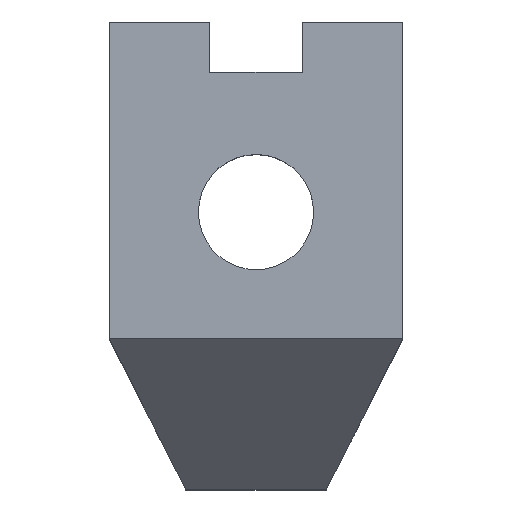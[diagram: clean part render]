
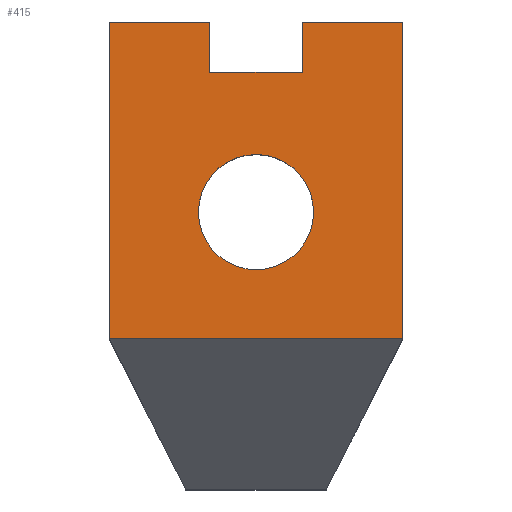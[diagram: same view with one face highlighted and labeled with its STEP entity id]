
A CAD part, top view. The second image highlights one B-rep face of the part: STEP entity #415.
In plain terms, the highlighted planar face has unit normal (0, 0, 1).
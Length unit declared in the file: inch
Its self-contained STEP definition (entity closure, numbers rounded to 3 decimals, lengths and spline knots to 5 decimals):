
#9 = VERTEX_POINT ( 'NONE', #203 ) ;
#13 = DIRECTION ( 'NONE',  ( 1., 0., 0. ) ) ;
#18 = CARTESIAN_POINT ( 'NONE',  ( 3., 1.675, 0.82 ) ) ;
#20 = CARTESIAN_POINT ( 'NONE',  ( 2.27004, 2.30413, 0.82 ) ) ;
#27 = ORIENTED_EDGE ( 'NONE', *, *, #751, .T. ) ;
#28 = VERTEX_POINT ( 'NONE', #416 ) ;
#43 = VERTEX_POINT ( 'NONE', #749 ) ;
#50 = VERTEX_POINT ( 'NONE', #125 ) ;
#52 = VERTEX_POINT ( 'NONE', #18 ) ;
#125 = CARTESIAN_POINT ( 'NONE',  ( 1.54, 1.675, 0.82 ) ) ;
#137 = CARTESIAN_POINT ( 'NONE',  ( 2.5, 3., 0.82 ) ) ;
#138 = VERTEX_POINT ( 'NONE', #782 ) ;
#164 = EDGE_LOOP ( 'NONE', ( #788, #383, #27, #991, #351, #967, #1031, #629 ) ) ;
#173 = CARTESIAN_POINT ( 'NONE',  ( 2.04, 3.25, 0.82 ) ) ;
#190 = VERTEX_POINT ( 'NONE', #1062 ) ;
#203 = CARTESIAN_POINT ( 'NONE',  ( 1.98343, 2.30413, 0.82 ) ) ;
#239 = DIRECTION ( 'NONE',  ( 0., 1., 0. ) ) ;
#243 = DIRECTION ( 'NONE',  ( 1., 0., 0. ) ) ;
#248 = CARTESIAN_POINT ( 'NONE',  ( 2.5, 3.25, 0.82 ) ) ;
#253 = CARTESIAN_POINT ( 'NONE',  ( 1.54, 1.675, 0.82 ) ) ;
#257 = CARTESIAN_POINT ( 'NONE',  ( 2.04, 3., 0.82 ) ) ;
#264 = DIRECTION ( 'NONE',  ( -1., 0., 0. ) ) ;
#281 = DIRECTION ( 'NONE',  ( 0., 0., -1. ) ) ;
#296 = DIRECTION ( 'NONE',  ( 0., 1., 0. ) ) ;
#334 = DIRECTION ( 'NONE',  ( -1., 0., 0. ) ) ;
#336 = CARTESIAN_POINT ( 'NONE',  ( 2.5, 3., 0.82 ) ) ;
#340 = DIRECTION ( 'NONE',  ( 0., -1., 0. ) ) ;
#342 = CARTESIAN_POINT ( 'NONE',  ( 1.54, 1.675, 0.82 ) ) ;
#346 = DIRECTION ( 'NONE',  ( 1., 0., 0. ) ) ;
#347 = DIRECTION ( 'NONE',  ( 0., 0., -1. ) ) ;
#348 = CARTESIAN_POINT ( 'NONE',  ( 2.27004, 2.30413, 0.82 ) ) ;
#351 = ORIENTED_EDGE ( 'NONE', *, *, #756, .T. ) ;
#353 = CARTESIAN_POINT ( 'NONE',  ( 3., 3.25, 0.82 ) ) ;
#354 = DIRECTION ( 'NONE',  ( 0., 0., 1. ) ) ;
#355 = CARTESIAN_POINT ( 'NONE',  ( 3., 3.25, 0.82 ) ) ;
#358 = DIRECTION ( 'NONE',  ( 0., -1., 0. ) ) ;
#363 = CARTESIAN_POINT ( 'NONE',  ( 2.04, 3., 0.82 ) ) ;
#373 = EDGE_LOOP ( 'NONE', ( #992, #1042 ) ) ;
#383 = ORIENTED_EDGE ( 'NONE', *, *, #750, .T. ) ;
#414 = FACE_BOUND ( 'NONE', #373, .T. ) ;
#415 = ADVANCED_FACE ( 'NONE', ( #937, #414 ), #570, .T. ) ;
#416 = CARTESIAN_POINT ( 'NONE',  ( 2.55665, 2.30413, 0.82 ) ) ;
#417 = DIRECTION ( 'NONE',  ( 1., 0., 0. ) ) ;
#436 = DIRECTION ( 'NONE',  ( 1., 0., 0. ) ) ;
#445 = CARTESIAN_POINT ( 'NONE',  ( 1.54, 3.25, 0.82 ) ) ;
#473 = AXIS2_PLACEMENT_3D ( 'NONE', #20, #281, #13 ) ;
#488 = VERTEX_POINT ( 'NONE', #173 ) ;
#552 = AXIS2_PLACEMENT_3D ( 'NONE', #348, #347, #346 ) ;
#570 = PLANE ( 'NONE',  #706 ) ;
#596 = CIRCLE ( 'NONE', #473, 0.28661 ) ;
#629 = ORIENTED_EDGE ( 'NONE', *, *, #761, .T. ) ;
#669 = CARTESIAN_POINT ( 'NONE',  ( 0., 0., 0.82 ) ) ;
#706 = AXIS2_PLACEMENT_3D ( 'NONE', #669, #354, #436 ) ;
#738 = VERTEX_POINT ( 'NONE', #363 ) ;
#743 = EDGE_CURVE ( 'NONE', #28, #9, #1055, .T. ) ;
#746 = EDGE_CURVE ( 'NONE', #190, #52, #1069, .T. ) ;
#749 = CARTESIAN_POINT ( 'NONE',  ( 2.5, 3.25, 0.82 ) ) ;
#750 = EDGE_CURVE ( 'NONE', #190, #43, #1039, .T. ) ;
#751 = EDGE_CURVE ( 'NONE', #43, #1047, #1037, .T. ) ;
#752 = EDGE_CURVE ( 'NONE', #1047, #738, #1025, .T. ) ;
#756 = EDGE_CURVE ( 'NONE', #738, #488, #1017, .T. ) ;
#758 = EDGE_CURVE ( 'NONE', #138, #488, #1015, .T. ) ;
#759 = EDGE_CURVE ( 'NONE', #50, #138, #1034, .T. ) ;
#761 = EDGE_CURVE ( 'NONE', #50, #52, #1009, .T. ) ;
#782 = CARTESIAN_POINT ( 'NONE',  ( 1.54, 3.25, 0.82 ) ) ;
#788 = ORIENTED_EDGE ( 'NONE', *, *, #746, .F. ) ;
#926 = EDGE_CURVE ( 'NONE', #9, #28, #596, .T. ) ;
#937 = FACE_OUTER_BOUND ( 'NONE', #164, .T. ) ;
#967 = ORIENTED_EDGE ( 'NONE', *, *, #758, .F. ) ;
#991 = ORIENTED_EDGE ( 'NONE', *, *, #752, .T. ) ;
#992 = ORIENTED_EDGE ( 'NONE', *, *, #926, .T. ) ;
#996 = VECTOR ( 'NONE', #243, 39.37008 ) ;
#998 = VECTOR ( 'NONE', #239, 39.37008 ) ;
#1008 = VECTOR ( 'NONE', #417, 39.37008 ) ;
#1009 = LINE ( 'NONE', #342, #996 ) ;
#1014 = VECTOR ( 'NONE', #296, 39.37008 ) ;
#1015 = LINE ( 'NONE', #445, #1008 ) ;
#1016 = VECTOR ( 'NONE', #334, 39.37008 ) ;
#1017 = LINE ( 'NONE', #257, #1014 ) ;
#1024 = VECTOR ( 'NONE', #340, 39.37008 ) ;
#1025 = LINE ( 'NONE', #336, #1016 ) ;
#1026 = VECTOR ( 'NONE', #264, 39.37008 ) ;
#1031 = ORIENTED_EDGE ( 'NONE', *, *, #759, .F. ) ;
#1034 = LINE ( 'NONE', #253, #998 ) ;
#1035 = VECTOR ( 'NONE', #358, 39.37008 ) ;
#1037 = LINE ( 'NONE', #248, #1024 ) ;
#1039 = LINE ( 'NONE', #355, #1026 ) ;
#1042 = ORIENTED_EDGE ( 'NONE', *, *, #743, .T. ) ;
#1047 = VERTEX_POINT ( 'NONE', #137 ) ;
#1055 = CIRCLE ( 'NONE', #552, 0.28661 ) ;
#1062 = CARTESIAN_POINT ( 'NONE',  ( 3., 3.25, 0.82 ) ) ;
#1069 = LINE ( 'NONE', #353, #1035 ) ;
